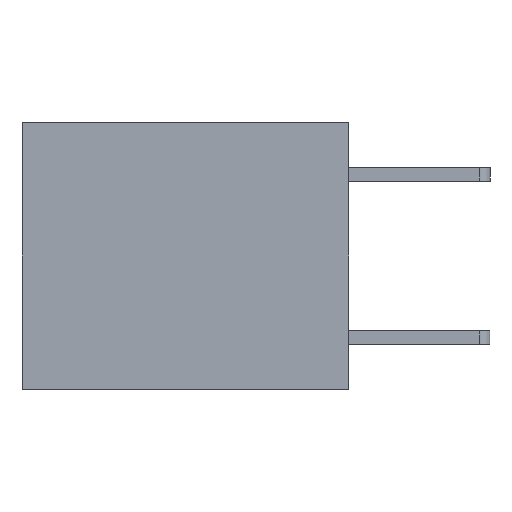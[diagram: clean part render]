
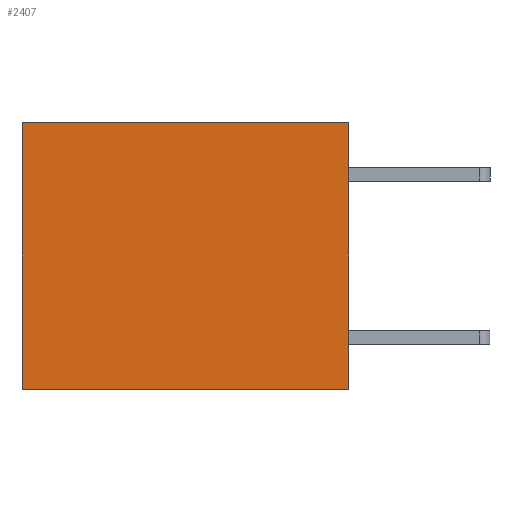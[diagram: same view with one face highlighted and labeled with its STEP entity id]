
A CAD part, left-side view. The second image highlights one B-rep face of the part: STEP entity #2407.
In plain terms, the highlighted planar face has unit normal (-1, 0, 0).
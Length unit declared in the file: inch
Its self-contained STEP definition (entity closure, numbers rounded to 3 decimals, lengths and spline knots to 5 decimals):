
#480 = EDGE_CURVE ( 'NONE', #2002, #8274, #8981, .T. ) ;
#619 = CARTESIAN_POINT ( 'NONE',  ( 0.3165, 0.6, -0.49 ) ) ;
#1017 = CARTESIAN_POINT ( 'NONE',  ( 0.3165, 0.6, 0. ) ) ;
#1139 = EDGE_CURVE ( 'NONE', #7061, #4899, #8116, .T. ) ;
#1164 = DIRECTION ( 'NONE',  ( 1., 0., 0. ) ) ;
#2002 = VERTEX_POINT ( 'NONE', #7626 ) ;
#2090 = ORIENTED_EDGE ( 'NONE', *, *, #480, .F. ) ;
#2407 = ADVANCED_FACE ( 'NONE', ( #5957 ), #3320, .F. ) ;
#2569 = CARTESIAN_POINT ( 'NONE',  ( 0.3165, 0., -0.49 ) ) ;
#2667 = EDGE_LOOP ( 'NONE', ( #6515, #2090, #5920, #4377 ) ) ;
#2770 = VECTOR ( 'NONE', #8296, 39.37008 ) ;
#3176 = DIRECTION ( 'NONE',  ( 0., 1., 0. ) ) ;
#3197 = VECTOR ( 'NONE', #3176, 39.37008 ) ;
#3320 = PLANE ( 'NONE',  #8147 ) ;
#4377 = ORIENTED_EDGE ( 'NONE', *, *, #1139, .T. ) ;
#4386 = DIRECTION ( 'NONE',  ( 0., 0., -1. ) ) ;
#4480 = EDGE_CURVE ( 'NONE', #7061, #2002, #5341, .T. ) ;
#4568 = VECTOR ( 'NONE', #4386, 39.37008 ) ;
#4747 = EDGE_CURVE ( 'NONE', #4899, #8274, #6728, .T. ) ;
#4899 = VERTEX_POINT ( 'NONE', #1017 ) ;
#5341 = LINE ( 'NONE', #2569, #2770 ) ;
#5563 = CARTESIAN_POINT ( 'NONE',  ( 0.3165, 0., 0. ) ) ;
#5614 = CARTESIAN_POINT ( 'NONE',  ( 0.3165, 0.6, -0.49 ) ) ;
#5920 = ORIENTED_EDGE ( 'NONE', *, *, #4480, .F. ) ;
#5957 = FACE_OUTER_BOUND ( 'NONE', #2667, .T. ) ;
#5960 = DIRECTION ( 'NONE',  ( 0., 1., 0. ) ) ;
#6151 = CARTESIAN_POINT ( 'NONE',  ( 0.3165, 0., -0.49 ) ) ;
#6186 = CARTESIAN_POINT ( 'NONE',  ( 0.3165, 0., -0.49 ) ) ;
#6198 = VECTOR ( 'NONE', #5960, 39.37008 ) ;
#6515 = ORIENTED_EDGE ( 'NONE', *, *, #4747, .T. ) ;
#6728 = LINE ( 'NONE', #619, #4568 ) ;
#6770 = CARTESIAN_POINT ( 'NONE',  ( 0.3165, 0., 0. ) ) ;
#7061 = VERTEX_POINT ( 'NONE', #5563 ) ;
#7626 = CARTESIAN_POINT ( 'NONE',  ( 0.3165, 0., -0.49 ) ) ;
#8116 = LINE ( 'NONE', #6770, #6198 ) ;
#8147 = AXIS2_PLACEMENT_3D ( 'NONE', #6151, #1164, #8210 ) ;
#8210 = DIRECTION ( 'NONE',  ( 0., 0., -1. ) ) ;
#8274 = VERTEX_POINT ( 'NONE', #5614 ) ;
#8296 = DIRECTION ( 'NONE',  ( 0., 0., -1. ) ) ;
#8981 = LINE ( 'NONE', #6186, #3197 ) ;
